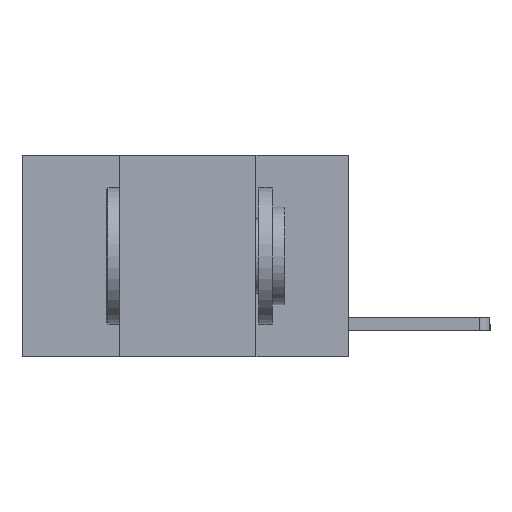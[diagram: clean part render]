
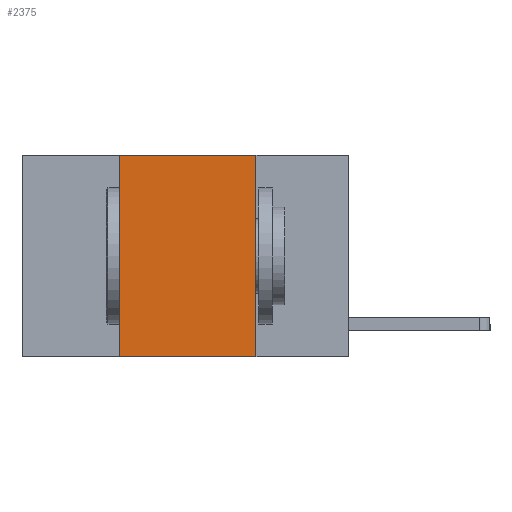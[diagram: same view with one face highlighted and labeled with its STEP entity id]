
A CAD part, left-side view. The second image highlights one B-rep face of the part: STEP entity #2375.
In plain terms, the highlighted planar face has unit normal (-1, 0, 0).
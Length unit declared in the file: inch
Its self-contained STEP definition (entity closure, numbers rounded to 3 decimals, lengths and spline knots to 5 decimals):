
#102 = ORIENTED_EDGE ( 'NONE', *, *, #649, .F. ) ;
#555 = VERTEX_POINT ( 'NONE', #1810 ) ;
#571 = LINE ( 'NONE', #4079, #1442 ) ;
#649 = EDGE_CURVE ( 'NONE', #555, #1910, #4364, .T. ) ;
#672 = CARTESIAN_POINT ( 'NONE',  ( 0., 0.6, 0. ) ) ;
#815 = VERTEX_POINT ( 'NONE', #10623 ) ;
#1442 = VECTOR ( 'NONE', #10920, 39.37008 ) ;
#1810 = CARTESIAN_POINT ( 'NONE',  ( 0., 0.42, -0.37 ) ) ;
#1910 = VERTEX_POINT ( 'NONE', #10946 ) ;
#2350 = VECTOR ( 'NONE', #9950, 39.37008 ) ;
#2375 = ADVANCED_FACE ( 'NONE', ( #3913 ), #7370, .F. ) ;
#2376 = EDGE_CURVE ( 'NONE', #815, #5840, #571, .T. ) ;
#2420 = EDGE_CURVE ( 'NONE', #1910, #815, #6484, .T. ) ;
#2534 = EDGE_CURVE ( 'NONE', #555, #5840, #8509, .T. ) ;
#3220 = CARTESIAN_POINT ( 'NONE',  ( 0., 0.6, 0. ) ) ;
#3913 = FACE_OUTER_BOUND ( 'NONE', #6773, .T. ) ;
#3991 = CARTESIAN_POINT ( 'NONE',  ( 0., 0.17, -0.37 ) ) ;
#4079 = CARTESIAN_POINT ( 'NONE',  ( 0., 0.17, 0. ) ) ;
#4364 = LINE ( 'NONE', #10510, #6028 ) ;
#4902 = VECTOR ( 'NONE', #11131, 39.37008 ) ;
#5427 = ORIENTED_EDGE ( 'NONE', *, *, #2420, .F. ) ;
#5623 = DIRECTION ( 'NONE',  ( 1., 0., 0. ) ) ;
#5840 = VERTEX_POINT ( 'NONE', #3991 ) ;
#6009 = ORIENTED_EDGE ( 'NONE', *, *, #2534, .T. ) ;
#6028 = VECTOR ( 'NONE', #7815, 39.37008 ) ;
#6121 = CARTESIAN_POINT ( 'NONE',  ( 0., 0.6, -0.37 ) ) ;
#6484 = LINE ( 'NONE', #3220, #2350 ) ;
#6510 = ORIENTED_EDGE ( 'NONE', *, *, #2376, .F. ) ;
#6698 = DIRECTION ( 'NONE',  ( 0., 0., -1. ) ) ;
#6773 = EDGE_LOOP ( 'NONE', ( #6510, #5427, #102, #6009 ) ) ;
#7370 = PLANE ( 'NONE',  #11244 ) ;
#7815 = DIRECTION ( 'NONE',  ( 0., 0., 1. ) ) ;
#8509 = LINE ( 'NONE', #6121, #4902 ) ;
#9950 = DIRECTION ( 'NONE',  ( 0., -1., 0. ) ) ;
#10510 = CARTESIAN_POINT ( 'NONE',  ( 0., 0.42, 0. ) ) ;
#10623 = CARTESIAN_POINT ( 'NONE',  ( 0., 0.17, 0. ) ) ;
#10920 = DIRECTION ( 'NONE',  ( 0., 0., -1. ) ) ;
#10946 = CARTESIAN_POINT ( 'NONE',  ( 0., 0.42, 0. ) ) ;
#11131 = DIRECTION ( 'NONE',  ( 0., -1., 0. ) ) ;
#11244 = AXIS2_PLACEMENT_3D ( 'NONE', #672, #5623, #6698 ) ;
